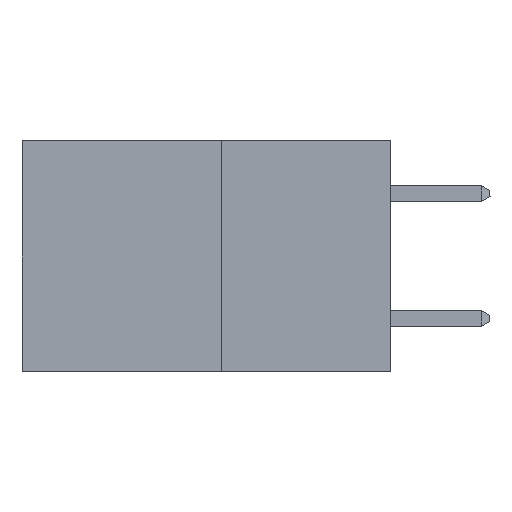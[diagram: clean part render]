
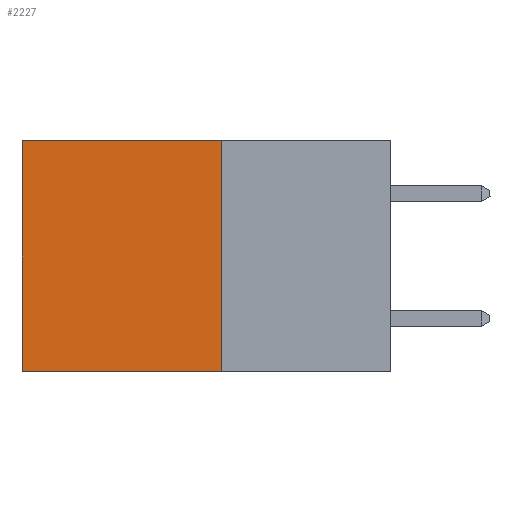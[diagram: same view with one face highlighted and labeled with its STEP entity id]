
A CAD part, left-side view. The second image highlights one B-rep face of the part: STEP entity #2227.
In plain terms, the highlighted planar face has unit normal (-1, 0, 0).
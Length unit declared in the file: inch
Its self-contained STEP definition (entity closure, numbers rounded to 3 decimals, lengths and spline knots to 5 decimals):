
#1212 = EDGE_CURVE ( 'NONE', #4837, #14138, #7935, .T. ) ;
#2227 = ADVANCED_FACE ( 'NONE', ( #9676 ), #7073, .F. ) ;
#2323 = CARTESIAN_POINT ( 'NONE',  ( 0.277, 0.27, -0.37 ) ) ;
#2761 = VECTOR ( 'NONE', #4615, 39.37008 ) ;
#4053 = EDGE_CURVE ( 'NONE', #4837, #8804, #9441, .T. ) ;
#4057 = LINE ( 'NONE', #4951, #6249 ) ;
#4567 = CARTESIAN_POINT ( 'NONE',  ( 0.277, 0.59, -0.37 ) ) ;
#4593 = CARTESIAN_POINT ( 'NONE',  ( 0.277, 0.27, -0.37 ) ) ;
#4615 = DIRECTION ( 'NONE',  ( 0., 0., -1. ) ) ;
#4837 = VERTEX_POINT ( 'NONE', #9072 ) ;
#4951 = CARTESIAN_POINT ( 'NONE',  ( 0.277, 0.27, -0.37 ) ) ;
#5005 = DIRECTION ( 'NONE',  ( 0., 1., 0. ) ) ;
#6068 = EDGE_CURVE ( 'NONE', #8804, #13896, #4057, .T. ) ;
#6249 = VECTOR ( 'NONE', #5005, 39.37008 ) ;
#6502 = ORIENTED_EDGE ( 'NONE', *, *, #1212, .T. ) ;
#6878 = ORIENTED_EDGE ( 'NONE', *, *, #7422, .T. ) ;
#7073 = PLANE ( 'NONE',  #12815 ) ;
#7307 = VECTOR ( 'NONE', #10793, 39.37008 ) ;
#7422 = EDGE_CURVE ( 'NONE', #14138, #13896, #13448, .T. ) ;
#7935 = LINE ( 'NONE', #14376, #11621 ) ;
#8061 = DIRECTION ( 'NONE',  ( 1., 0., 0. ) ) ;
#8169 = CARTESIAN_POINT ( 'NONE',  ( 0.277, 0.59, -0.37 ) ) ;
#8804 = VERTEX_POINT ( 'NONE', #10504 ) ;
#9072 = CARTESIAN_POINT ( 'NONE',  ( 0.277, 0.27, 0. ) ) ;
#9441 = LINE ( 'NONE', #4593, #2761 ) ;
#9676 = FACE_OUTER_BOUND ( 'NONE', #11545, .T. ) ;
#10157 = DIRECTION ( 'NONE',  ( 0., 0., -1. ) ) ;
#10504 = CARTESIAN_POINT ( 'NONE',  ( 0.277, 0.27, -0.37 ) ) ;
#10793 = DIRECTION ( 'NONE',  ( 0., 0., -1. ) ) ;
#11342 = ORIENTED_EDGE ( 'NONE', *, *, #4053, .F. ) ;
#11545 = EDGE_LOOP ( 'NONE', ( #6878, #13803, #11342, #6502 ) ) ;
#11621 = VECTOR ( 'NONE', #13783, 39.37008 ) ;
#12815 = AXIS2_PLACEMENT_3D ( 'NONE', #2323, #8061, #10157 ) ;
#13428 = CARTESIAN_POINT ( 'NONE',  ( 0.277, 0.59, 0. ) ) ;
#13448 = LINE ( 'NONE', #4567, #7307 ) ;
#13783 = DIRECTION ( 'NONE',  ( 0., 1., 0. ) ) ;
#13803 = ORIENTED_EDGE ( 'NONE', *, *, #6068, .F. ) ;
#13896 = VERTEX_POINT ( 'NONE', #8169 ) ;
#14138 = VERTEX_POINT ( 'NONE', #13428 ) ;
#14376 = CARTESIAN_POINT ( 'NONE',  ( 0.277, 0.27, 0. ) ) ;
